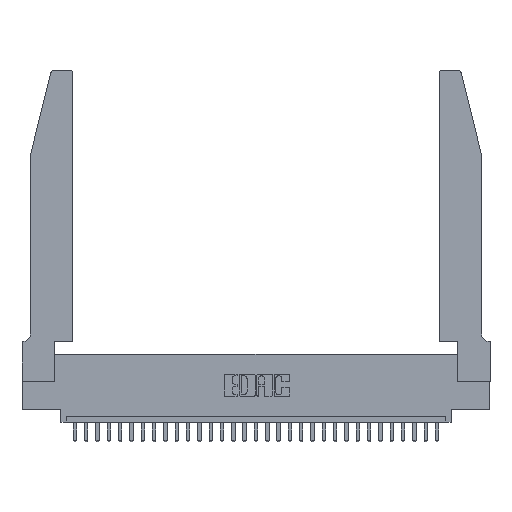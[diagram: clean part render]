
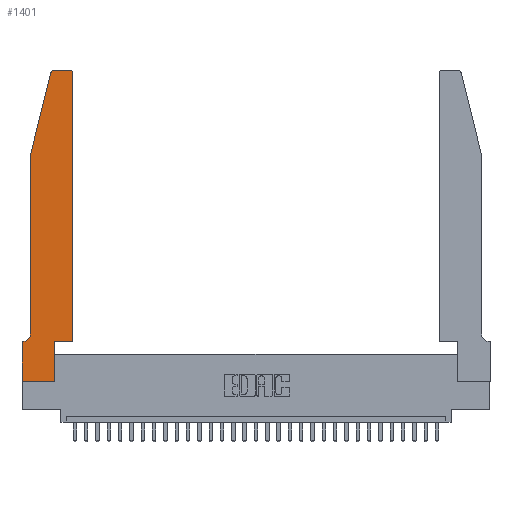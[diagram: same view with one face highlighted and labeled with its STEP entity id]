
A CAD part, top view. The second image highlights one B-rep face of the part: STEP entity #1401.
In plain terms, the highlighted planar face has unit normal (0, 0, 1).
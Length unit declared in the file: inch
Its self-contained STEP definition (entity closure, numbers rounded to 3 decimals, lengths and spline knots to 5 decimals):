
#550 = DIRECTION ( 'NONE',  ( 1., 0., 0. ) ) ;
#849 = CARTESIAN_POINT ( 'NONE',  ( 0.0755, 2., 0.37 ) ) ;
#1401 = ADVANCED_FACE ( 'NONE', ( #8865 ), #19804, .T. ) ;
#1662 = ORIENTED_EDGE ( 'NONE', *, *, #7587, .T. ) ;
#1940 = ORIENTED_EDGE ( 'NONE', *, *, #10022, .T. ) ;
#2032 = CARTESIAN_POINT ( 'NONE',  ( 0.2865, 0., 0.37 ) ) ;
#2229 = EDGE_CURVE ( 'NONE', #16801, #25360, #27537, .T. ) ;
#2626 = VERTEX_POINT ( 'NONE', #30941 ) ;
#3740 = AXIS2_PLACEMENT_3D ( 'NONE', #16215, #23343, #6028 ) ;
#3890 = CARTESIAN_POINT ( 'NONE',  ( 0.4505, 0.35, 0.37 ) ) ;
#5304 = DIRECTION ( 'NONE',  ( 0., 0., -1. ) ) ;
#5387 = ORIENTED_EDGE ( 'NONE', *, *, #10266, .T. ) ;
#5432 = ORIENTED_EDGE ( 'NONE', *, *, #10672, .T. ) ;
#5688 = DIRECTION ( 'NONE',  ( 0., 0., 1. ) ) ;
#5769 = ORIENTED_EDGE ( 'NONE', *, *, #12226, .T. ) ;
#5802 = VECTOR ( 'NONE', #27040, 39.37008 ) ;
#5941 = CARTESIAN_POINT ( 'NONE',  ( 0.4205, 2.75, 0.37 ) ) ;
#5952 = AXIS2_PLACEMENT_3D ( 'NONE', #6506, #5688, #18694 ) ;
#6028 = DIRECTION ( 'NONE',  ( 1., 0., 0. ) ) ;
#6205 = VECTOR ( 'NONE', #14367, 39.37008 ) ;
#6506 = CARTESIAN_POINT ( 'NONE',  ( 0.4205, 2.72, 0.37 ) ) ;
#6528 = ORIENTED_EDGE ( 'NONE', *, *, #24734, .T. ) ;
#6611 = AXIS2_PLACEMENT_3D ( 'NONE', #28822, #5304, #19566 ) ;
#7587 = EDGE_CURVE ( 'NONE', #27247, #2626, #13342, .T. ) ;
#7920 = CIRCLE ( 'NONE', #3740, 0.03 ) ;
#7978 = VERTEX_POINT ( 'NONE', #20095 ) ;
#8055 = EDGE_CURVE ( 'NONE', #8445, #24943, #15177, .T. ) ;
#8445 = VERTEX_POINT ( 'NONE', #27749 ) ;
#8625 = LINE ( 'NONE', #15832, #19096 ) ;
#8865 = FACE_OUTER_BOUND ( 'NONE', #17359, .T. ) ;
#9411 = CARTESIAN_POINT ( 'NONE',  ( 0.4505, 2.72, 0.37 ) ) ;
#10022 = EDGE_CURVE ( 'NONE', #18066, #25263, #27477, .T. ) ;
#10266 = EDGE_CURVE ( 'NONE', #27531, #16801, #16972, .T. ) ;
#10323 = VECTOR ( 'NONE', #28483, 39.37008 ) ;
#10672 = EDGE_CURVE ( 'NONE', #25360, #14875, #7920, .T. ) ;
#11760 = EDGE_CURVE ( 'NONE', #27598, #27531, #8625, .T. ) ;
#12226 = EDGE_CURVE ( 'NONE', #24943, #27247, #14347, .T. ) ;
#12685 = CARTESIAN_POINT ( 'NONE',  ( 0., 0., 0.37 ) ) ;
#13033 = CARTESIAN_POINT ( 'NONE',  ( 0., 0., 0.37 ) ) ;
#13342 = LINE ( 'NONE', #27462, #16369 ) ;
#14347 = CIRCLE ( 'NONE', #6611, 0.07 ) ;
#14367 = DIRECTION ( 'NONE',  ( -0.239, -0.971, 0. ) ) ;
#14489 = DIRECTION ( 'NONE',  ( 1., 0., 0. ) ) ;
#14804 = CARTESIAN_POINT ( 'NONE',  ( 0., 0.35, 0.37 ) ) ;
#14875 = VERTEX_POINT ( 'NONE', #19236 ) ;
#15177 = LINE ( 'NONE', #849, #5802 ) ;
#15832 = CARTESIAN_POINT ( 'NONE',  ( 0.4505, 0.35, 0.37 ) ) ;
#16113 = CARTESIAN_POINT ( 'NONE',  ( 0.2865, 0.35, 0.37 ) ) ;
#16215 = CARTESIAN_POINT ( 'NONE',  ( 0.284, 2.72, 0.37 ) ) ;
#16369 = VECTOR ( 'NONE', #24711, 39.37008 ) ;
#16452 = EDGE_CURVE ( 'NONE', #14875, #8445, #29098, .T. ) ;
#16787 = CARTESIAN_POINT ( 'NONE',  ( 0.284, 2.75, 0.37 ) ) ;
#16801 = VERTEX_POINT ( 'NONE', #5941 ) ;
#16835 = LINE ( 'NONE', #3890, #28849 ) ;
#16972 = CIRCLE ( 'NONE', #5952, 0.03 ) ;
#17309 = DIRECTION ( 'NONE',  ( 0., -1., 0. ) ) ;
#17359 = EDGE_LOOP ( 'NONE', ( #24336, #5432, #23099, #19814, #5769, #1662, #24736, #1940, #6528, #30191, #30945, #5387 ) ) ;
#17639 = CARTESIAN_POINT ( 'NONE',  ( 0.0755, 0.42, 0.37 ) ) ;
#18066 = VERTEX_POINT ( 'NONE', #13033 ) ;
#18148 = VECTOR ( 'NONE', #17309, 39.37008 ) ;
#18694 = DIRECTION ( 'NONE',  ( 1., 0., 0. ) ) ;
#19096 = VECTOR ( 'NONE', #25604, 39.37008 ) ;
#19220 = DIRECTION ( 'NONE',  ( 1., 0., 0. ) ) ;
#19236 = CARTESIAN_POINT ( 'NONE',  ( 0.25487, 2.72718, 0.37 ) ) ;
#19284 = VECTOR ( 'NONE', #19348, 39.37008 ) ;
#19348 = DIRECTION ( 'NONE',  ( -1., 0., 0. ) ) ;
#19566 = DIRECTION ( 'NONE',  ( -1., 0., 0. ) ) ;
#19804 = PLANE ( 'NONE',  #27375 ) ;
#19814 = ORIENTED_EDGE ( 'NONE', *, *, #8055, .T. ) ;
#20095 = CARTESIAN_POINT ( 'NONE',  ( 0.2865, 0.35, 0.37 ) ) ;
#21874 = CARTESIAN_POINT ( 'NONE',  ( 0.2605, 2.75, 0.37 ) ) ;
#22242 = VECTOR ( 'NONE', #19220, 39.37008 ) ;
#23099 = ORIENTED_EDGE ( 'NONE', *, *, #16452, .T. ) ;
#23343 = DIRECTION ( 'NONE',  ( 0., 0., 1. ) ) ;
#23836 = LINE ( 'NONE', #16113, #10323 ) ;
#23858 = CARTESIAN_POINT ( 'NONE',  ( 0.4505, 0.35, 0.37 ) ) ;
#23886 = CARTESIAN_POINT ( 'NONE',  ( 0.0755, 2., 0.37 ) ) ;
#24228 = DIRECTION ( 'NONE',  ( 0., 0., 1. ) ) ;
#24336 = ORIENTED_EDGE ( 'NONE', *, *, #2229, .T. ) ;
#24711 = DIRECTION ( 'NONE',  ( -1., 0., 0. ) ) ;
#24734 = EDGE_CURVE ( 'NONE', #25263, #7978, #23836, .T. ) ;
#24736 = ORIENTED_EDGE ( 'NONE', *, *, #26593, .T. ) ;
#24929 = CARTESIAN_POINT ( 'NONE',  ( 0.0055, 0.35, 0.37 ) ) ;
#24943 = VERTEX_POINT ( 'NONE', #17639 ) ;
#25263 = VERTEX_POINT ( 'NONE', #2032 ) ;
#25360 = VERTEX_POINT ( 'NONE', #16787 ) ;
#25604 = DIRECTION ( 'NONE',  ( 0., 1., 0. ) ) ;
#26593 = EDGE_CURVE ( 'NONE', #2626, #18066, #30910, .T. ) ;
#27040 = DIRECTION ( 'NONE',  ( 0., -1., 0. ) ) ;
#27247 = VERTEX_POINT ( 'NONE', #24929 ) ;
#27375 = AXIS2_PLACEMENT_3D ( 'NONE', #14804, #24228, #550 ) ;
#27462 = CARTESIAN_POINT ( 'NONE',  ( 0.0755, 0.35, 0.37 ) ) ;
#27477 = LINE ( 'NONE', #28671, #22242 ) ;
#27531 = VERTEX_POINT ( 'NONE', #9411 ) ;
#27537 = LINE ( 'NONE', #21874, #19284 ) ;
#27598 = VERTEX_POINT ( 'NONE', #23858 ) ;
#27749 = CARTESIAN_POINT ( 'NONE',  ( 0.0755, 2., 0.37 ) ) ;
#28483 = DIRECTION ( 'NONE',  ( 0., 1., 0. ) ) ;
#28671 = CARTESIAN_POINT ( 'NONE',  ( 0., 0., 0.37 ) ) ;
#28822 = CARTESIAN_POINT ( 'NONE',  ( 0.0055, 0.42, 0.37 ) ) ;
#28849 = VECTOR ( 'NONE', #14489, 39.37008 ) ;
#29098 = LINE ( 'NONE', #23886, #6205 ) ;
#30023 = EDGE_CURVE ( 'NONE', #7978, #27598, #16835, .T. ) ;
#30191 = ORIENTED_EDGE ( 'NONE', *, *, #30023, .T. ) ;
#30910 = LINE ( 'NONE', #12685, #18148 ) ;
#30941 = CARTESIAN_POINT ( 'NONE',  ( 0., 0.35, 0.37 ) ) ;
#30945 = ORIENTED_EDGE ( 'NONE', *, *, #11760, .T. ) ;
